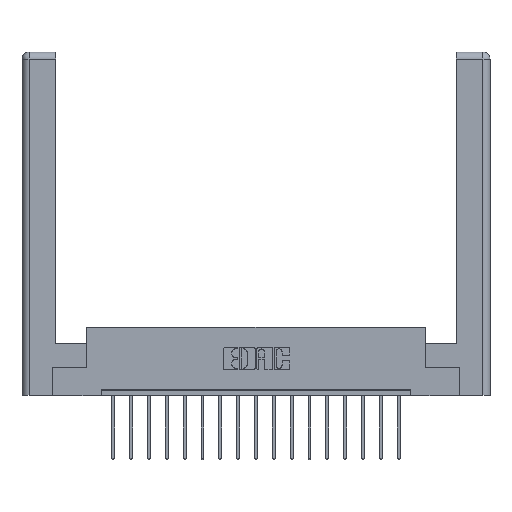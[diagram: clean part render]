
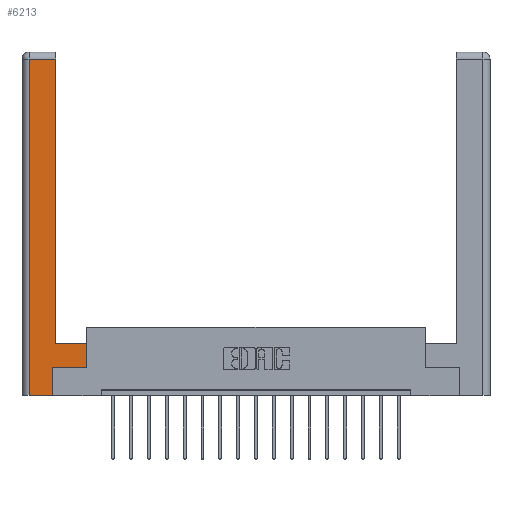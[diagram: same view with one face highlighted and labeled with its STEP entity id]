
A CAD part, top view. The second image highlights one B-rep face of the part: STEP entity #6213.
In plain terms, the highlighted planar face has unit normal (0, 0, 1).
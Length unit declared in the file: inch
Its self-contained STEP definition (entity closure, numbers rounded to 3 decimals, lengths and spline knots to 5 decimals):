
#67 = VERTEX_POINT ( 'NONE', #11221 ) ;
#70 = EDGE_CURVE ( 'NONE', #3271, #67, #9996, .T. ) ;
#161 = FACE_OUTER_BOUND ( 'NONE', #13633, .T. ) ;
#347 = CARTESIAN_POINT ( 'NONE',  ( 0.0615, 0., 0. ) ) ;
#354 = VERTEX_POINT ( 'NONE', #9410 ) ;
#574 = CARTESIAN_POINT ( 'NONE',  ( 0.565, 0.45, 0. ) ) ;
#883 = ORIENTED_EDGE ( 'NONE', *, *, #14880, .T. ) ;
#1231 = DIRECTION ( 'NONE',  ( -1., 0., 0. ) ) ;
#1632 = VECTOR ( 'NONE', #1231, 39.37008 ) ;
#1704 = EDGE_CURVE ( 'NONE', #10164, #354, #16461, .T. ) ;
#1758 = VECTOR ( 'NONE', #10061, 39.37008 ) ;
#1787 = DIRECTION ( 'NONE',  ( 0., -1., 0. ) ) ;
#2077 = DIRECTION ( 'NONE',  ( 1., 0., 0. ) ) ;
#2376 = PLANE ( 'NONE',  #16232 ) ;
#3271 = VERTEX_POINT ( 'NONE', #7575 ) ;
#3307 = CARTESIAN_POINT ( 'NONE',  ( 0.295, 2.94, 0. ) ) ;
#3496 = ORIENTED_EDGE ( 'NONE', *, *, #1704, .T. ) ;
#3668 = LINE ( 'NONE', #11192, #10149 ) ;
#3813 = LINE ( 'NONE', #11218, #8501 ) ;
#4719 = ORIENTED_EDGE ( 'NONE', *, *, #7658, .T. ) ;
#4743 = CARTESIAN_POINT ( 'NONE',  ( 0.0615, 2.94, 0. ) ) ;
#5248 = VECTOR ( 'NONE', #2077, 39.37008 ) ;
#5360 = ORIENTED_EDGE ( 'NONE', *, *, #70, .T. ) ;
#6047 = VERTEX_POINT ( 'NONE', #3307 ) ;
#6213 = ADVANCED_FACE ( 'NONE', ( #161 ), #2376, .F. ) ;
#6507 = ORIENTED_EDGE ( 'NONE', *, *, #11458, .T. ) ;
#7095 = DIRECTION ( 'NONE',  ( 0., 1., 0. ) ) ;
#7575 = CARTESIAN_POINT ( 'NONE',  ( 0.265, 0.245, 0. ) ) ;
#7658 = EDGE_CURVE ( 'NONE', #354, #6047, #3668, .T. ) ;
#7984 = ORIENTED_EDGE ( 'NONE', *, *, #8344, .T. ) ;
#8043 = CARTESIAN_POINT ( 'NONE',  ( 0.295, 0.45, 0. ) ) ;
#8057 = ORIENTED_EDGE ( 'NONE', *, *, #9773, .T. ) ;
#8098 = DIRECTION ( 'NONE',  ( -1., 0., 0. ) ) ;
#8344 = EDGE_CURVE ( 'NONE', #15633, #18426, #18215, .T. ) ;
#8425 = DIRECTION ( 'NONE',  ( -1., 0., 0. ) ) ;
#8501 = VECTOR ( 'NONE', #14068, 39.37008 ) ;
#8786 = VECTOR ( 'NONE', #1787, 39.37008 ) ;
#9248 = CARTESIAN_POINT ( 'NONE',  ( 0.0615, 0., 0. ) ) ;
#9410 = CARTESIAN_POINT ( 'NONE',  ( 0.295, 0.45, 0. ) ) ;
#9610 = ORIENTED_EDGE ( 'NONE', *, *, #14835, .T. ) ;
#9773 = EDGE_CURVE ( 'NONE', #10450, #3271, #3813, .T. ) ;
#9996 = LINE ( 'NONE', #18544, #1758 ) ;
#10061 = DIRECTION ( 'NONE',  ( 1., 0., 0. ) ) ;
#10149 = VECTOR ( 'NONE', #7095, 39.37008 ) ;
#10164 = VERTEX_POINT ( 'NONE', #13536 ) ;
#10450 = VERTEX_POINT ( 'NONE', #11961 ) ;
#10535 = LINE ( 'NONE', #16924, #1632 ) ;
#10715 = DIRECTION ( 'NONE',  ( 0., 0., -1. ) ) ;
#10719 = DIRECTION ( 'NONE',  ( 0., 1., 0. ) ) ;
#11192 = CARTESIAN_POINT ( 'NONE',  ( 0.295, 3., 0. ) ) ;
#11218 = CARTESIAN_POINT ( 'NONE',  ( 0.265, 0.245, 0. ) ) ;
#11221 = CARTESIAN_POINT ( 'NONE',  ( 0.565, 0.245, 0. ) ) ;
#11458 = EDGE_CURVE ( 'NONE', #6047, #15633, #10535, .T. ) ;
#11471 = VECTOR ( 'NONE', #8425, 39.37008 ) ;
#11961 = CARTESIAN_POINT ( 'NONE',  ( 0.265, 0., 0. ) ) ;
#12410 = LINE ( 'NONE', #16475, #5248 ) ;
#13323 = VECTOR ( 'NONE', #10719, 39.37008 ) ;
#13536 = CARTESIAN_POINT ( 'NONE',  ( 0.565, 0.45, 0. ) ) ;
#13547 = LINE ( 'NONE', #574, #13323 ) ;
#13633 = EDGE_LOOP ( 'NONE', ( #4719, #6507, #7984, #883, #8057, #5360, #9610, #3496 ) ) ;
#14068 = DIRECTION ( 'NONE',  ( 0., 1., 0. ) ) ;
#14835 = EDGE_CURVE ( 'NONE', #67, #10164, #13547, .T. ) ;
#14880 = EDGE_CURVE ( 'NONE', #18426, #10450, #12410, .T. ) ;
#15633 = VERTEX_POINT ( 'NONE', #4743 ) ;
#16232 = AXIS2_PLACEMENT_3D ( 'NONE', #16720, #10715, #8098 ) ;
#16461 = LINE ( 'NONE', #8043, #11471 ) ;
#16475 = CARTESIAN_POINT ( 'NONE',  ( 0.265, 0., 0. ) ) ;
#16720 = CARTESIAN_POINT ( 'NONE',  ( 0., 0., 0. ) ) ;
#16924 = CARTESIAN_POINT ( 'NONE',  ( 0.0615, 2.94, 0. ) ) ;
#18215 = LINE ( 'NONE', #347, #8786 ) ;
#18426 = VERTEX_POINT ( 'NONE', #9248 ) ;
#18544 = CARTESIAN_POINT ( 'NONE',  ( 0.565, 0.245, 0. ) ) ;
